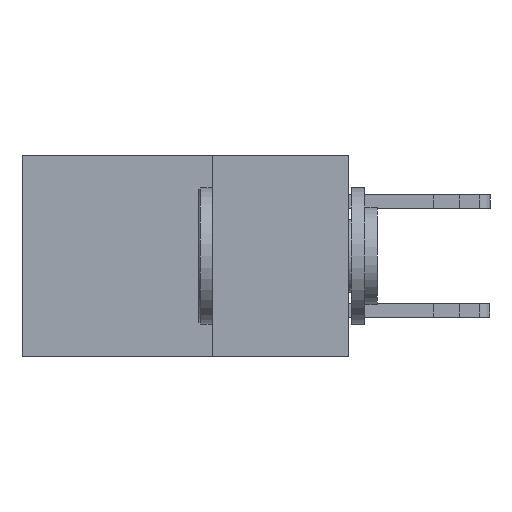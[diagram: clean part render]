
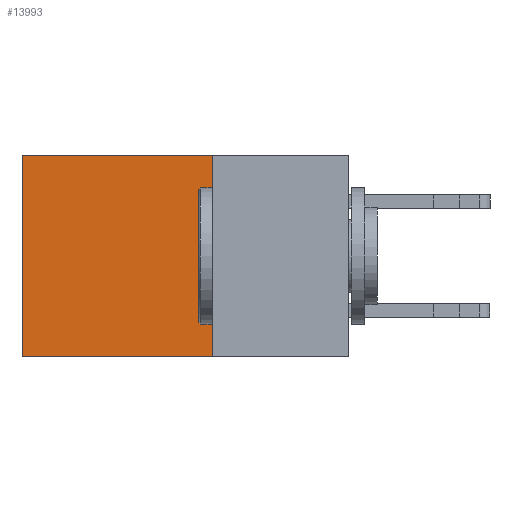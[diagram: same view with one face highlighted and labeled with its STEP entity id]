
A CAD part, left-side view. The second image highlights one B-rep face of the part: STEP entity #13993.
In plain terms, the highlighted planar face has unit normal (-1, 0, 0).
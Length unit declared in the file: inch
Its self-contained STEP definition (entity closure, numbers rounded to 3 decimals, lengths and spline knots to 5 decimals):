
#152 = ORIENTED_EDGE ( 'NONE', *, *, #10303, .F. ) ;
#1374 = FACE_OUTER_BOUND ( 'NONE', #9136, .T. ) ;
#1503 = VECTOR ( 'NONE', #6113, 39.37008 ) ;
#1583 = LINE ( 'NONE', #7489, #5467 ) ;
#2048 = VECTOR ( 'NONE', #12313, 39.37008 ) ;
#3008 = CARTESIAN_POINT ( 'NONE',  ( 0.298, 0.25, -0.37 ) ) ;
#3745 = VECTOR ( 'NONE', #15021, 39.37008 ) ;
#3966 = EDGE_CURVE ( 'NONE', #8319, #11805, #5549, .T. ) ;
#4638 = CARTESIAN_POINT ( 'NONE',  ( 0.298, 0.25, 0. ) ) ;
#5439 = CARTESIAN_POINT ( 'NONE',  ( 0.298, 0.6, 0. ) ) ;
#5467 = VECTOR ( 'NONE', #8668, 39.37008 ) ;
#5549 = LINE ( 'NONE', #11774, #2048 ) ;
#5700 = CARTESIAN_POINT ( 'NONE',  ( 0.298, 0.6, -0.37 ) ) ;
#5812 = DIRECTION ( 'NONE',  ( 1., 0., 0. ) ) ;
#6113 = DIRECTION ( 'NONE',  ( 0., 0., -1. ) ) ;
#7042 = CARTESIAN_POINT ( 'NONE',  ( 0.298, 0.25, -0.37 ) ) ;
#7208 = LINE ( 'NONE', #7042, #3745 ) ;
#7489 = CARTESIAN_POINT ( 'NONE',  ( 0.298, 0.6, 0. ) ) ;
#7930 = ORIENTED_EDGE ( 'NONE', *, *, #10160, .F. ) ;
#8113 = LINE ( 'NONE', #10692, #1503 ) ;
#8319 = VERTEX_POINT ( 'NONE', #13091 ) ;
#8463 = ORIENTED_EDGE ( 'NONE', *, *, #13755, .T. ) ;
#8668 = DIRECTION ( 'NONE',  ( 0., 0., -1. ) ) ;
#9136 = EDGE_LOOP ( 'NONE', ( #8463, #7930, #152, #14551 ) ) ;
#10160 = EDGE_CURVE ( 'NONE', #13204, #11392, #7208, .T. ) ;
#10303 = EDGE_CURVE ( 'NONE', #8319, #13204, #8113, .T. ) ;
#10692 = CARTESIAN_POINT ( 'NONE',  ( 0.298, 0.25, 0. ) ) ;
#11392 = VERTEX_POINT ( 'NONE', #5700 ) ;
#11774 = CARTESIAN_POINT ( 'NONE',  ( 0.298, 0.25, 0. ) ) ;
#11805 = VERTEX_POINT ( 'NONE', #5439 ) ;
#12271 = AXIS2_PLACEMENT_3D ( 'NONE', #4638, #5812, #13844 ) ;
#12313 = DIRECTION ( 'NONE',  ( 0., 1., 0. ) ) ;
#12690 = PLANE ( 'NONE',  #12271 ) ;
#13091 = CARTESIAN_POINT ( 'NONE',  ( 0.298, 0.25, 0. ) ) ;
#13204 = VERTEX_POINT ( 'NONE', #3008 ) ;
#13755 = EDGE_CURVE ( 'NONE', #11805, #11392, #1583, .T. ) ;
#13844 = DIRECTION ( 'NONE',  ( 0., 0., -1. ) ) ;
#13993 = ADVANCED_FACE ( 'NONE', ( #1374 ), #12690, .F. ) ;
#14551 = ORIENTED_EDGE ( 'NONE', *, *, #3966, .T. ) ;
#15021 = DIRECTION ( 'NONE',  ( 0., 1., 0. ) ) ;
